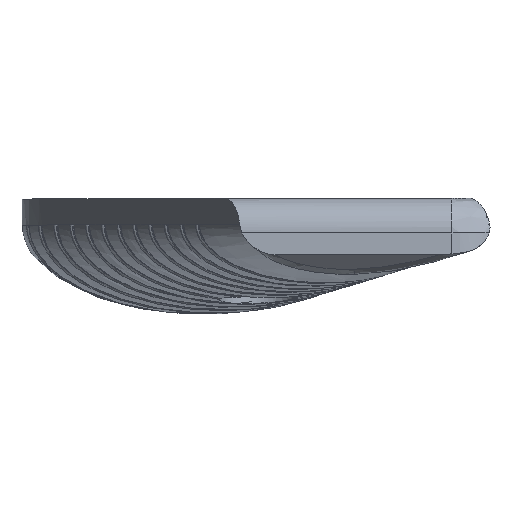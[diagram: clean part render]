
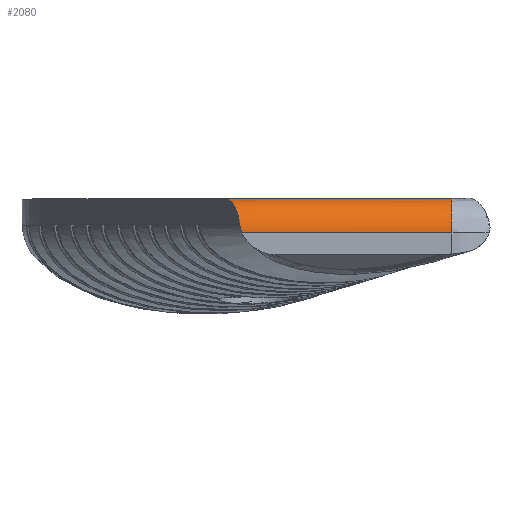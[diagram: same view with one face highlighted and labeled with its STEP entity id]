
A CAD part, top view. The second image highlights one B-rep face of the part: STEP entity #2080.
In plain terms, the highlighted cylindrical face has radius 4 mm (diameter 8 mm), a partial arc.
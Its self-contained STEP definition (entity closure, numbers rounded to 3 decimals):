
#101=CIRCLE('',#2121,4.);
#318=B_SPLINE_CURVE_WITH_KNOTS('',3,(#21331,#21332,#21333,#21334,#21335,
#21336,#21337,#21338,#21339,#21340),.UNSPECIFIED.,.F.,.F.,(4,2,2,2,4),(0.,
0.009,0.021,0.029,0.039),
 .UNSPECIFIED.);
#321=B_SPLINE_CURVE_WITH_KNOTS('',3,(#21542,#21543,#21544,#21545,#21546,
#21547,#21548,#21549,#21550,#21551,#21552,#21553,#21554,#21555,#21556,#21557),
 .UNSPECIFIED.,.F.,.F.,(4,2,2,2,2,2,2,4),(0.,0.006,
0.014,0.032,0.141,0.287,
0.428,0.561),.UNSPECIFIED.);
#483=FACE_OUTER_BOUND('',#613,.T.);
#613=EDGE_LOOP('',(#1880,#1881,#1882,#1883,#1884));
#670=LINE('',#2495,#739);
#677=LINE('',#18953,#746);
#739=VECTOR('',#2240,1000.);
#746=VECTOR('',#2325,1000.);
#804=VERTEX_POINT('',#2492);
#805=VERTEX_POINT('',#2494);
#819=VERTEX_POINT('',#2692);
#978=VERTEX_POINT('',#18952);
#981=VERTEX_POINT('',#21330);
#1013=EDGE_CURVE('',#805,#804,#670,.T.);
#1031=EDGE_CURVE('',#819,#805,#101,.T.);
#1245=EDGE_CURVE('',#978,#819,#677,.T.);
#1293=EDGE_CURVE('',#981,#978,#318,.T.);
#1301=EDGE_CURVE('',#804,#981,#321,.T.);
#1880=ORIENTED_EDGE('',*,*,#1013,.T.);
#1881=ORIENTED_EDGE('',*,*,#1301,.T.);
#1882=ORIENTED_EDGE('',*,*,#1293,.T.);
#1883=ORIENTED_EDGE('',*,*,#1245,.T.);
#1884=ORIENTED_EDGE('',*,*,#1031,.T.);
#1956=CYLINDRICAL_SURFACE('',#2178,4.);
#2080=ADVANCED_FACE('',(#483),#1956,.T.);
#2121=AXIS2_PLACEMENT_3D('',#2693,#2256,#2257);
#2178=AXIS2_PLACEMENT_3D('',#21541,#2409,#2410);
#2240=DIRECTION('',(-1.,0.,0.));
#2256=DIRECTION('center_axis',(-1.,0.,0.));
#2257=DIRECTION('ref_axis',(0.,0.,1.));
#2325=DIRECTION('',(1.,0.,0.));
#2409=DIRECTION('center_axis',(-1.,0.,0.));
#2410=DIRECTION('ref_axis',(0.,1.,0.));
#2492=CARTESIAN_POINT('',(-37.278,-36.861,8.277));
#2494=CARTESIAN_POINT('',(-11.058,-36.862,8.277));
#2495=CARTESIAN_POINT('',(-24.247,-36.861,8.277));
#2692=CARTESIAN_POINT('',(-11.058,-40.862,12.277));
#2693=CARTESIAN_POINT('Origin',(-11.058,-40.862,8.277));
#18952=CARTESIAN_POINT('',(-35.236,-40.861,12.277));
#18953=CARTESIAN_POINT('',(-24.247,-40.861,12.277));
#21330=CARTESIAN_POINT('',(-35.489,-39.861,12.15));
#21331=CARTESIAN_POINT('Ctrl Pts',(-35.489,-39.861,12.15));
#21332=CARTESIAN_POINT('Ctrl Pts',(-35.485,-39.89,
12.157));
#21333=CARTESIAN_POINT('Ctrl Pts',(-35.481,-39.951,
12.173));
#21334=CARTESIAN_POINT('Ctrl Pts',(-35.453,-40.146,
12.214));
#21335=CARTESIAN_POINT('Ctrl Pts',(-35.43,-40.259,
12.233));
#21336=CARTESIAN_POINT('Ctrl Pts',(-35.384,-40.445,
12.256));
#21337=CARTESIAN_POINT('Ctrl Pts',(-35.361,-40.521,
12.263));
#21338=CARTESIAN_POINT('Ctrl Pts',(-35.307,-40.686,
12.274));
#21339=CARTESIAN_POINT('Ctrl Pts',(-35.273,-40.774,
12.277));
#21340=CARTESIAN_POINT('Ctrl Pts',(-35.236,-40.861,
12.277));
#21541=CARTESIAN_POINT('Origin',(-11.058,-40.862,8.277));
#21542=CARTESIAN_POINT('Ctrl Pts',(-37.278,-36.861,
8.277));
#21543=CARTESIAN_POINT('Ctrl Pts',(-37.269,-36.861,
8.296));
#21544=CARTESIAN_POINT('Ctrl Pts',(-37.26,-36.861,
8.315));
#21545=CARTESIAN_POINT('Ctrl Pts',(-37.24,-36.862,
8.358));
#21546=CARTESIAN_POINT('Ctrl Pts',(-37.229,-36.862,8.382));
#21547=CARTESIAN_POINT('Ctrl Pts',(-37.193,-36.865,
8.461));
#21548=CARTESIAN_POINT('Ctrl Pts',(-37.167,-36.868,
8.516));
#21549=CARTESIAN_POINT('Ctrl Pts',(-36.991,-36.896,
8.899));
#21550=CARTESIAN_POINT('Ctrl Pts',(-36.84,-36.961,
9.224));
#21551=CARTESIAN_POINT('Ctrl Pts',(-36.499,-37.206,
9.962));
#21552=CARTESIAN_POINT('Ctrl Pts',(-36.313,-37.419,
10.364));
#21553=CARTESIAN_POINT('Ctrl Pts',(-35.985,-37.969,
11.075));
#21554=CARTESIAN_POINT('Ctrl Pts',(-35.843,-38.299,
11.382));
#21555=CARTESIAN_POINT('Ctrl Pts',(-35.621,-39.039,11.863));
#21556=CARTESIAN_POINT('Ctrl Pts',(-35.539,-39.437,
12.04));
#21557=CARTESIAN_POINT('Ctrl Pts',(-35.489,-39.861,
12.15));
